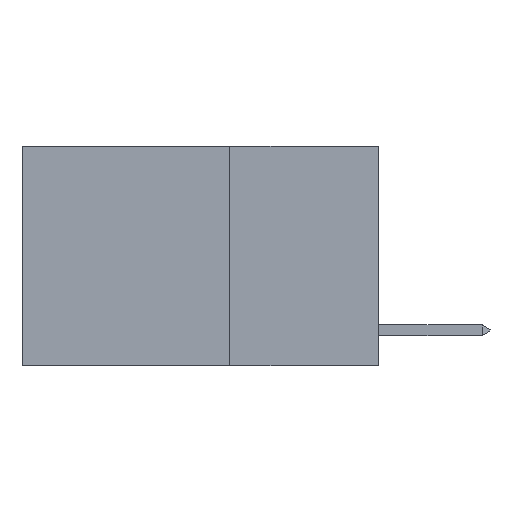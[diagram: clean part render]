
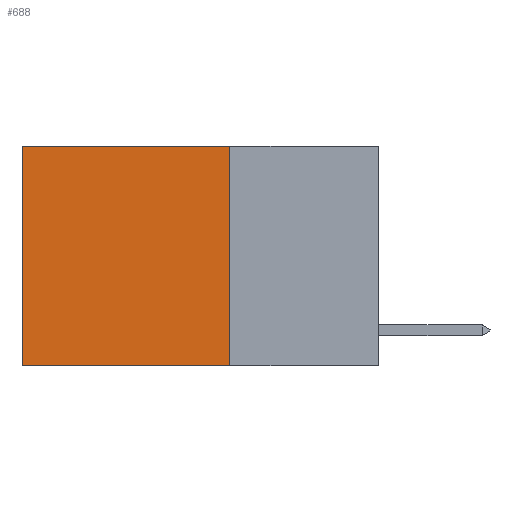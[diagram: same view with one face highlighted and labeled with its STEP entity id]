
A CAD part, left-side view. The second image highlights one B-rep face of the part: STEP entity #688.
In plain terms, the highlighted planar face has unit normal (-1, 0, 0).
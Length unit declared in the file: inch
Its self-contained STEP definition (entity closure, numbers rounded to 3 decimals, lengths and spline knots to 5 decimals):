
#672 = VERTEX_POINT ( 'NONE', #9489 ) ;
#688 = ADVANCED_FACE ( 'NONE', ( #10621 ), #14084, .F. ) ;
#1687 = CARTESIAN_POINT ( 'NONE',  ( 0.2625, 0.6, 0. ) ) ;
#1806 = ORIENTED_EDGE ( 'NONE', *, *, #4509, .T. ) ;
#2152 = EDGE_CURVE ( 'NONE', #672, #12812, #12651, .T. ) ;
#2712 = VECTOR ( 'NONE', #4008, 39.37008 ) ;
#3620 = CARTESIAN_POINT ( 'NONE',  ( 0.2625, 0.25, -0.37 ) ) ;
#3882 = LINE ( 'NONE', #1687, #2712 ) ;
#3909 = CARTESIAN_POINT ( 'NONE',  ( 0.2625, 0.6, -0.37 ) ) ;
#4008 = DIRECTION ( 'NONE',  ( 0., 0., -1. ) ) ;
#4043 = VECTOR ( 'NONE', #13765, 39.37008 ) ;
#4067 = CARTESIAN_POINT ( 'NONE',  ( 0.2625, 0.25, 0. ) ) ;
#4509 = EDGE_CURVE ( 'NONE', #672, #5358, #6546, .T. ) ;
#4527 = CARTESIAN_POINT ( 'NONE',  ( 0.2625, 0.6, 0. ) ) ;
#4641 = AXIS2_PLACEMENT_3D ( 'NONE', #4067, #11523, #8583 ) ;
#4749 = VERTEX_POINT ( 'NONE', #3909 ) ;
#4918 = VECTOR ( 'NONE', #13827, 39.37008 ) ;
#5358 = VERTEX_POINT ( 'NONE', #4527 ) ;
#5906 = ORIENTED_EDGE ( 'NONE', *, *, #2152, .F. ) ;
#6546 = LINE ( 'NONE', #8946, #11249 ) ;
#6560 = EDGE_LOOP ( 'NONE', ( #9477, #8118, #5906, #1806 ) ) ;
#7034 = EDGE_CURVE ( 'NONE', #5358, #4749, #3882, .T. ) ;
#7756 = CARTESIAN_POINT ( 'NONE',  ( 0.2625, 0.25, -0.37 ) ) ;
#8118 = ORIENTED_EDGE ( 'NONE', *, *, #13636, .F. ) ;
#8583 = DIRECTION ( 'NONE',  ( 0., 0., -1. ) ) ;
#8946 = CARTESIAN_POINT ( 'NONE',  ( 0.2625, 0.25, 0. ) ) ;
#9477 = ORIENTED_EDGE ( 'NONE', *, *, #7034, .T. ) ;
#9489 = CARTESIAN_POINT ( 'NONE',  ( 0.2625, 0.25, 0. ) ) ;
#10621 = FACE_OUTER_BOUND ( 'NONE', #6560, .T. ) ;
#11249 = VECTOR ( 'NONE', #13477, 39.37008 ) ;
#11523 = DIRECTION ( 'NONE',  ( 1., 0., 0. ) ) ;
#12651 = LINE ( 'NONE', #12871, #4918 ) ;
#12659 = LINE ( 'NONE', #3620, #4043 ) ;
#12812 = VERTEX_POINT ( 'NONE', #7756 ) ;
#12871 = CARTESIAN_POINT ( 'NONE',  ( 0.2625, 0.25, 0. ) ) ;
#13477 = DIRECTION ( 'NONE',  ( 0., 1., 0. ) ) ;
#13636 = EDGE_CURVE ( 'NONE', #12812, #4749, #12659, .T. ) ;
#13765 = DIRECTION ( 'NONE',  ( 0., 1., 0. ) ) ;
#13827 = DIRECTION ( 'NONE',  ( 0., 0., -1. ) ) ;
#14084 = PLANE ( 'NONE',  #4641 ) ;
